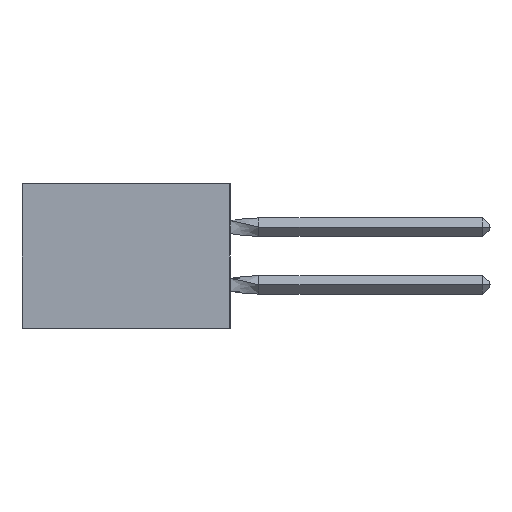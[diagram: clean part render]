
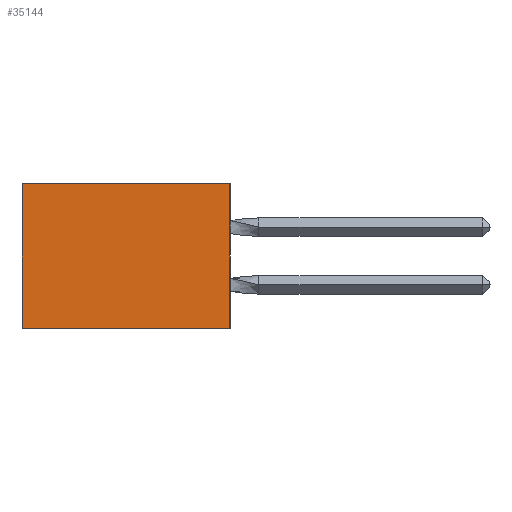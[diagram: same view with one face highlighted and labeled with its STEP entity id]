
A CAD part, left-side view. The second image highlights one B-rep face of the part: STEP entity #35144.
In plain terms, the highlighted planar face has unit normal (-1, 0, 0).
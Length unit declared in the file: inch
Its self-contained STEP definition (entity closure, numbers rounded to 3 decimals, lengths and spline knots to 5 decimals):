
#575 = CARTESIAN_POINT ( 'NONE',  ( 0.305, 0.72, -0.5 ) ) ;
#1528 = AXIS2_PLACEMENT_3D ( 'NONE', #37243, #19424, #25584 ) ;
#1709 = CARTESIAN_POINT ( 'NONE',  ( 0.305, 0., 0. ) ) ;
#2269 = EDGE_LOOP ( 'NONE', ( #5145, #4661, #8292, #3968 ) ) ;
#2776 = DIRECTION ( 'NONE',  ( 0., 1., 0. ) ) ;
#2785 = CARTESIAN_POINT ( 'NONE',  ( 0.305, 0.72, -0.5 ) ) ;
#3169 = VERTEX_POINT ( 'NONE', #25587 ) ;
#3968 = ORIENTED_EDGE ( 'NONE', *, *, #5599, .T. ) ;
#4661 = ORIENTED_EDGE ( 'NONE', *, *, #5663, .F. ) ;
#5145 = ORIENTED_EDGE ( 'NONE', *, *, #35495, .T. ) ;
#5599 = EDGE_CURVE ( 'NONE', #3169, #22151, #11457, .T. ) ;
#5663 = EDGE_CURVE ( 'NONE', #30658, #24916, #9637, .T. ) ;
#8191 = LINE ( 'NONE', #19094, #14134 ) ;
#8292 = ORIENTED_EDGE ( 'NONE', *, *, #10194, .F. ) ;
#9637 = LINE ( 'NONE', #29464, #26108 ) ;
#10194 = EDGE_CURVE ( 'NONE', #3169, #30658, #8191, .T. ) ;
#11457 = LINE ( 'NONE', #1709, #13296 ) ;
#13296 = VECTOR ( 'NONE', #36795, 39.37008 ) ;
#14134 = VECTOR ( 'NONE', #22156, 39.37008 ) ;
#17506 = FACE_OUTER_BOUND ( 'NONE', #2269, .T. ) ;
#19094 = CARTESIAN_POINT ( 'NONE',  ( 0.305, 0., -0.5 ) ) ;
#19424 = DIRECTION ( 'NONE',  ( 1., 0., 0. ) ) ;
#22151 = VERTEX_POINT ( 'NONE', #31695 ) ;
#22156 = DIRECTION ( 'NONE',  ( 0., 0., -1. ) ) ;
#24916 = VERTEX_POINT ( 'NONE', #2785 ) ;
#25584 = DIRECTION ( 'NONE',  ( 0., 0., -1. ) ) ;
#25587 = CARTESIAN_POINT ( 'NONE',  ( 0.305, 0., 0. ) ) ;
#26108 = VECTOR ( 'NONE', #2776, 39.37008 ) ;
#27011 = CARTESIAN_POINT ( 'NONE',  ( 0.305, 0., -0.5 ) ) ;
#28051 = LINE ( 'NONE', #575, #30368 ) ;
#29464 = CARTESIAN_POINT ( 'NONE',  ( 0.305, 0., -0.5 ) ) ;
#30368 = VECTOR ( 'NONE', #32951, 39.37008 ) ;
#30658 = VERTEX_POINT ( 'NONE', #27011 ) ;
#31695 = CARTESIAN_POINT ( 'NONE',  ( 0.305, 0.72, 0. ) ) ;
#32951 = DIRECTION ( 'NONE',  ( 0., 0., -1. ) ) ;
#35144 = ADVANCED_FACE ( 'NONE', ( #17506 ), #37121, .F. ) ;
#35495 = EDGE_CURVE ( 'NONE', #22151, #24916, #28051, .T. ) ;
#36795 = DIRECTION ( 'NONE',  ( 0., 1., 0. ) ) ;
#37121 = PLANE ( 'NONE',  #1528 ) ;
#37243 = CARTESIAN_POINT ( 'NONE',  ( 0.305, 0., -0.5 ) ) ;
